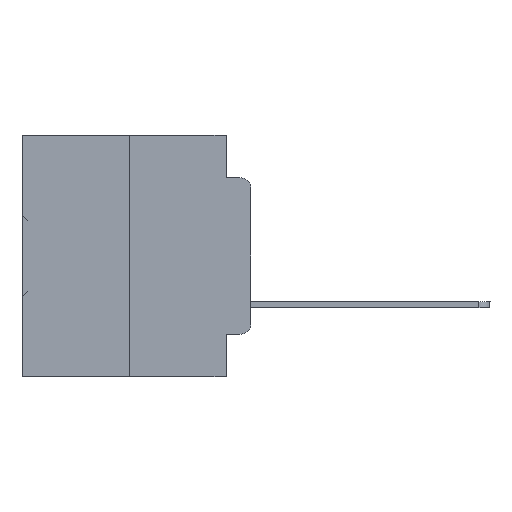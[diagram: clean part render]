
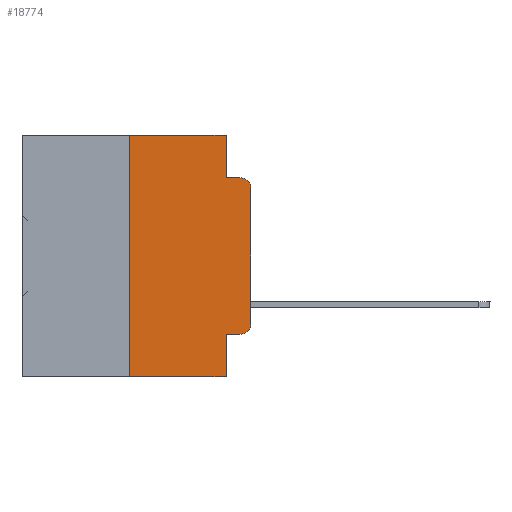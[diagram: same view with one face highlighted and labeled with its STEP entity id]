
A CAD part, left-side view. The second image highlights one B-rep face of the part: STEP entity #18774.
In plain terms, the highlighted planar face has unit normal (-1, 0, 0).
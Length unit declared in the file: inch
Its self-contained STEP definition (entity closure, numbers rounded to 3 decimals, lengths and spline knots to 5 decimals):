
#740 = EDGE_CURVE ( 'NONE', #30687, #15169, #11589, .T. ) ;
#1329 = CARTESIAN_POINT ( 'NONE',  ( 0., 0.02, -0.4115 ) ) ;
#1506 = EDGE_LOOP ( 'NONE', ( #30491, #14716, #25924, #6082, #4752, #22179, #5538, #21588, #13225, #16453 ) ) ;
#1854 = DIRECTION ( 'NONE',  ( 0., 0., 1. ) ) ;
#2156 = DIRECTION ( 'NONE',  ( 0., 0., -1. ) ) ;
#2478 = AXIS2_PLACEMENT_3D ( 'NONE', #20133, #23183, #2156 ) ;
#2541 = CARTESIAN_POINT ( 'NONE',  ( 0., 0.473, 0. ) ) ;
#2583 = DIRECTION ( 'NONE',  ( 0., -1., 0. ) ) ;
#2673 = LINE ( 'NONE', #37248, #32127 ) ;
#2795 = VERTEX_POINT ( 'NONE', #17301 ) ;
#2919 = CARTESIAN_POINT ( 'NONE',  ( 0., 0.051, -0.5 ) ) ;
#2947 = CARTESIAN_POINT ( 'NONE',  ( 0., 0.02, -0.0885 ) ) ;
#3099 = CIRCLE ( 'NONE', #37615, 0.02 ) ;
#3573 = EDGE_CURVE ( 'NONE', #27871, #13768, #21775, .T. ) ;
#3583 = PLANE ( 'NONE',  #28250 ) ;
#3684 = CARTESIAN_POINT ( 'NONE',  ( 0., 0.051, -0.4115 ) ) ;
#4752 = ORIENTED_EDGE ( 'NONE', *, *, #7295, .F. ) ;
#5538 = ORIENTED_EDGE ( 'NONE', *, *, #12166, .T. ) ;
#5718 = LINE ( 'NONE', #2541, #38028 ) ;
#5907 = EDGE_CURVE ( 'NONE', #32767, #21831, #22602, .T. ) ;
#6049 = DIRECTION ( 'NONE',  ( -1., 0., 0. ) ) ;
#6082 = ORIENTED_EDGE ( 'NONE', *, *, #26282, .F. ) ;
#6769 = EDGE_CURVE ( 'NONE', #26702, #24387, #13445, .T. ) ;
#7048 = CARTESIAN_POINT ( 'NONE',  ( 0., 0.473, 0. ) ) ;
#7295 = EDGE_CURVE ( 'NONE', #13768, #2795, #5718, .T. ) ;
#7727 = CARTESIAN_POINT ( 'NONE',  ( 0., 0.051, 0. ) ) ;
#8684 = CARTESIAN_POINT ( 'NONE',  ( 0., 0., -0.1085 ) ) ;
#9090 = DIRECTION ( 'NONE',  ( 0., -1., 0. ) ) ;
#11417 = CARTESIAN_POINT ( 'NONE',  ( 0., 0.25, 0. ) ) ;
#11589 = LINE ( 'NONE', #27311, #14475 ) ;
#11614 = CARTESIAN_POINT ( 'NONE',  ( 0., 0., -0.3915 ) ) ;
#11637 = CIRCLE ( 'NONE', #2478, 0.02 ) ;
#12166 = EDGE_CURVE ( 'NONE', #27871, #13261, #2673, .T. ) ;
#13225 = ORIENTED_EDGE ( 'NONE', *, *, #6769, .T. ) ;
#13261 = VERTEX_POINT ( 'NONE', #2919 ) ;
#13445 = LINE ( 'NONE', #33122, #27666 ) ;
#13768 = VERTEX_POINT ( 'NONE', #11417 ) ;
#14475 = VECTOR ( 'NONE', #9090, 39.37008 ) ;
#14716 = ORIENTED_EDGE ( 'NONE', *, *, #32681, .T. ) ;
#14955 = DIRECTION ( 'NONE',  ( 0., -1., 0. ) ) ;
#15169 = VERTEX_POINT ( 'NONE', #2947 ) ;
#16453 = ORIENTED_EDGE ( 'NONE', *, *, #29418, .T. ) ;
#17301 = CARTESIAN_POINT ( 'NONE',  ( 0., 0.051, 0. ) ) ;
#18550 = DIRECTION ( 'NONE',  ( 0., 0., -1. ) ) ;
#18774 = ADVANCED_FACE ( 'NONE', ( #28659 ), #3583, .F. ) ;
#20133 = CARTESIAN_POINT ( 'NONE',  ( 0., 0.02, -0.1085 ) ) ;
#20345 = CARTESIAN_POINT ( 'NONE',  ( 0., 0., 0. ) ) ;
#20379 = LINE ( 'NONE', #20701, #35097 ) ;
#20701 = CARTESIAN_POINT ( 'NONE',  ( 0., 0.051, 0. ) ) ;
#21405 = VECTOR ( 'NONE', #25981, 39.37008 ) ;
#21588 = ORIENTED_EDGE ( 'NONE', *, *, #27101, .F. ) ;
#21758 = DIRECTION ( 'NONE',  ( 0., -1., 0. ) ) ;
#21775 = LINE ( 'NONE', #30334, #22734 ) ;
#21831 = VERTEX_POINT ( 'NONE', #8684 ) ;
#22179 = ORIENTED_EDGE ( 'NONE', *, *, #3573, .F. ) ;
#22602 = LINE ( 'NONE', #20345, #29689 ) ;
#22734 = VECTOR ( 'NONE', #33523, 39.37008 ) ;
#23183 = DIRECTION ( 'NONE',  ( -1., 0., 0. ) ) ;
#23316 = LINE ( 'NONE', #7727, #21405 ) ;
#24387 = VERTEX_POINT ( 'NONE', #1329 ) ;
#24840 = CARTESIAN_POINT ( 'NONE',  ( 0., 0.02, -0.3915 ) ) ;
#25924 = ORIENTED_EDGE ( 'NONE', *, *, #740, .F. ) ;
#25981 = DIRECTION ( 'NONE',  ( 0., 0., -1. ) ) ;
#26282 = EDGE_CURVE ( 'NONE', #2795, #30687, #23316, .T. ) ;
#26702 = VERTEX_POINT ( 'NONE', #3684 ) ;
#27101 = EDGE_CURVE ( 'NONE', #26702, #13261, #20379, .T. ) ;
#27311 = CARTESIAN_POINT ( 'NONE',  ( 0., 0.051, -0.0885 ) ) ;
#27666 = VECTOR ( 'NONE', #2583, 39.37008 ) ;
#27871 = VERTEX_POINT ( 'NONE', #36822 ) ;
#28250 = AXIS2_PLACEMENT_3D ( 'NONE', #7048, #34277, #34410 ) ;
#28659 = FACE_OUTER_BOUND ( 'NONE', #1506, .T. ) ;
#29418 = EDGE_CURVE ( 'NONE', #24387, #32767, #3099, .T. ) ;
#29689 = VECTOR ( 'NONE', #1854, 39.37008 ) ;
#30334 = CARTESIAN_POINT ( 'NONE',  ( 0., 0.25, 0. ) ) ;
#30491 = ORIENTED_EDGE ( 'NONE', *, *, #5907, .T. ) ;
#30687 = VERTEX_POINT ( 'NONE', #31632 ) ;
#31632 = CARTESIAN_POINT ( 'NONE',  ( 0., 0.051, -0.0885 ) ) ;
#32127 = VECTOR ( 'NONE', #21758, 39.37008 ) ;
#32681 = EDGE_CURVE ( 'NONE', #21831, #15169, #11637, .T. ) ;
#32767 = VERTEX_POINT ( 'NONE', #11614 ) ;
#33122 = CARTESIAN_POINT ( 'NONE',  ( 0., 0.051, -0.4115 ) ) ;
#33523 = DIRECTION ( 'NONE',  ( 0., 0., 1. ) ) ;
#34277 = DIRECTION ( 'NONE',  ( 1., 0., 0. ) ) ;
#34410 = DIRECTION ( 'NONE',  ( 0., 0., -1. ) ) ;
#35097 = VECTOR ( 'NONE', #39244, 39.37008 ) ;
#36822 = CARTESIAN_POINT ( 'NONE',  ( 0., 0.25, -0.5 ) ) ;
#37248 = CARTESIAN_POINT ( 'NONE',  ( 0., 0.473, -0.5 ) ) ;
#37615 = AXIS2_PLACEMENT_3D ( 'NONE', #24840, #6049, #18550 ) ;
#38028 = VECTOR ( 'NONE', #14955, 39.37008 ) ;
#39244 = DIRECTION ( 'NONE',  ( 0., 0., -1. ) ) ;
